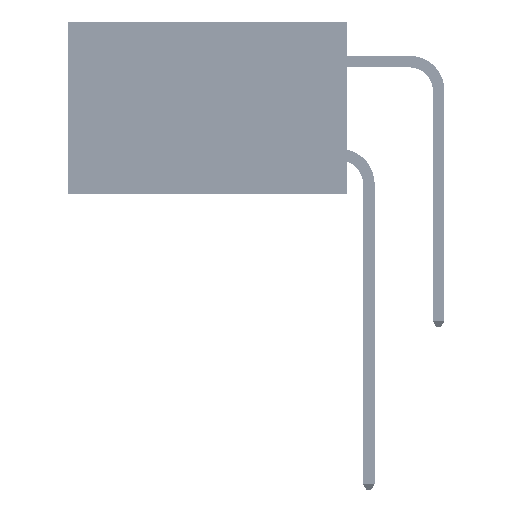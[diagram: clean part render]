
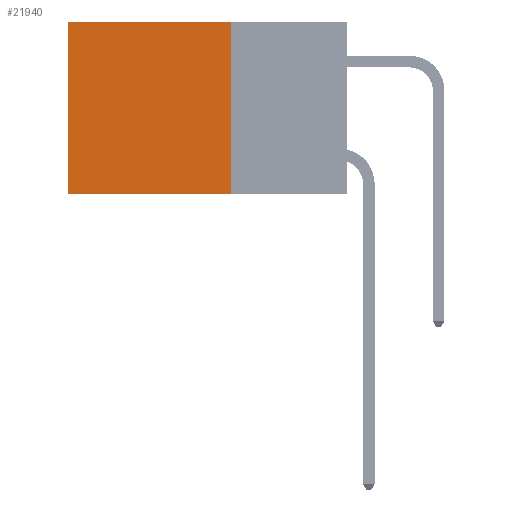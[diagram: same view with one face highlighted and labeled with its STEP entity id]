
A CAD part, left-side view. The second image highlights one B-rep face of the part: STEP entity #21940.
In plain terms, the highlighted planar face has unit normal (-1, 0, 0).
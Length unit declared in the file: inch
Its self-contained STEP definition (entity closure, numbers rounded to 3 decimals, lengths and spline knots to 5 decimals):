
#238 = CARTESIAN_POINT ( 'NONE',  ( 0.2875, 0.25, 0. ) ) ;
#1376 = LINE ( 'NONE', #16667, #8127 ) ;
#4740 = EDGE_CURVE ( 'NONE', #26917, #13762, #29992, .T. ) ;
#6009 = CARTESIAN_POINT ( 'NONE',  ( 0.2875, 0.6, -0.37 ) ) ;
#7011 = EDGE_CURVE ( 'NONE', #10679, #13762, #36552, .T. ) ;
#8127 = VECTOR ( 'NONE', #24926, 39.37008 ) ;
#9600 = DIRECTION ( 'NONE',  ( 0., 0., -1. ) ) ;
#10031 = DIRECTION ( 'NONE',  ( 0., 0., -1. ) ) ;
#10679 = VERTEX_POINT ( 'NONE', #15087 ) ;
#11836 = AXIS2_PLACEMENT_3D ( 'NONE', #36805, #13275, #10031 ) ;
#13178 = EDGE_CURVE ( 'NONE', #43092, #26917, #50760, .T. ) ;
#13275 = DIRECTION ( 'NONE',  ( 1., 0., 0. ) ) ;
#13762 = VERTEX_POINT ( 'NONE', #6009 ) ;
#15087 = CARTESIAN_POINT ( 'NONE',  ( 0.2875, 0.6, 0. ) ) ;
#16667 = CARTESIAN_POINT ( 'NONE',  ( 0.2875, 0.25, 0. ) ) ;
#17735 = FACE_OUTER_BOUND ( 'NONE', #19750, .T. ) ;
#19529 = VECTOR ( 'NONE', #28133, 39.37008 ) ;
#19750 = EDGE_LOOP ( 'NONE', ( #32876, #35054, #26451, #34863 ) ) ;
#19760 = CARTESIAN_POINT ( 'NONE',  ( 0.2875, 0.25, 0. ) ) ;
#19869 = CARTESIAN_POINT ( 'NONE',  ( 0.2875, 0.25, -0.37 ) ) ;
#21940 = ADVANCED_FACE ( 'NONE', ( #17735 ), #32982, .F. ) ;
#24926 = DIRECTION ( 'NONE',  ( 0., 1., 0. ) ) ;
#26451 = ORIENTED_EDGE ( 'NONE', *, *, #13178, .F. ) ;
#26917 = VERTEX_POINT ( 'NONE', #50176 ) ;
#28133 = DIRECTION ( 'NONE',  ( 0., 1., 0. ) ) ;
#29992 = LINE ( 'NONE', #19869, #19529 ) ;
#31637 = VECTOR ( 'NONE', #39744, 39.37008 ) ;
#32876 = ORIENTED_EDGE ( 'NONE', *, *, #7011, .T. ) ;
#32982 = PLANE ( 'NONE',  #11836 ) ;
#34863 = ORIENTED_EDGE ( 'NONE', *, *, #44625, .T. ) ;
#35054 = ORIENTED_EDGE ( 'NONE', *, *, #4740, .F. ) ;
#36552 = LINE ( 'NONE', #44644, #42660 ) ;
#36805 = CARTESIAN_POINT ( 'NONE',  ( 0.2875, 0.25, 0. ) ) ;
#39744 = DIRECTION ( 'NONE',  ( 0., 0., -1. ) ) ;
#42660 = VECTOR ( 'NONE', #9600, 39.37008 ) ;
#43092 = VERTEX_POINT ( 'NONE', #19760 ) ;
#44625 = EDGE_CURVE ( 'NONE', #43092, #10679, #1376, .T. ) ;
#44644 = CARTESIAN_POINT ( 'NONE',  ( 0.2875, 0.6, 0. ) ) ;
#50176 = CARTESIAN_POINT ( 'NONE',  ( 0.2875, 0.25, -0.37 ) ) ;
#50760 = LINE ( 'NONE', #238, #31637 ) ;
